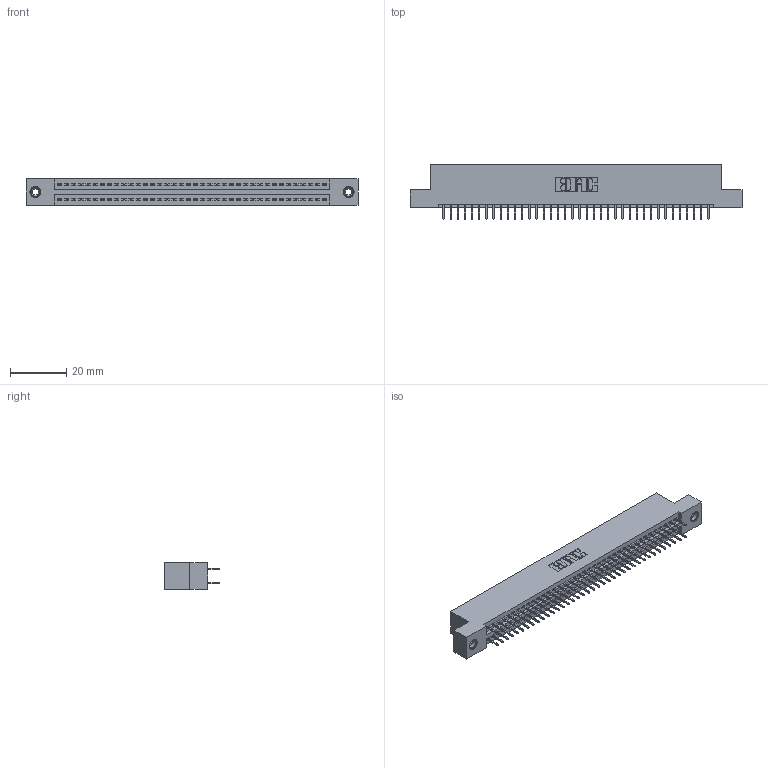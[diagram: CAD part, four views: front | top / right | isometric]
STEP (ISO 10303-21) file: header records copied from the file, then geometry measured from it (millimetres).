
FILE_DESCRIPTION (( 'STEP AP203' ), '1' );
FILE_NAME ('395-076-524-208.STEP', '2018-11-27T21:02:57', ( '' ), ( '' ), 'SwSTEP 2.0', 'SolidWorks 2016', '' );
FILE_SCHEMA (( 'CONFIG_CONTROL_DESIGN' ));
Length unit declared in the file: inch
Products named in the file (4): 345-250-001_345-250-003-102; 345-292-001_345-293-124; 345 Part_Flush Mounting Lugs - 0.156 Dia-TI; 395-076-524-208
Assembly tree (79 placements, depth 2):
  395-076-524-208
    345 Part_Flush Mounting Lugs - 0.156 Dia-TI
    345-292-001_345-293-124  x76
    345-250-001_345-250-003-102  x2
Bounding box: 117.73 x 19.35 x 9.4 mm (x, y, z)
Volume: 11277.7 mm3; surface area: 16302.6 mm2
Topology: 79 solids, 79 shells, 4290 faces, 12105 edges, 7758 vertices
Faces by surface type: plane 3076, cylinder 1198, cone 12, torus 4
Entity records: 31614 total; most frequent: CARTESIAN_POINT 5283, ORIENTED_EDGE 5210, DIRECTION 4691, EDGE_CURVE 2605, LINE 2305, VECTOR 2305, VERTEX_POINT 1728, AXIS2_PLACEMENT_3D 1193
